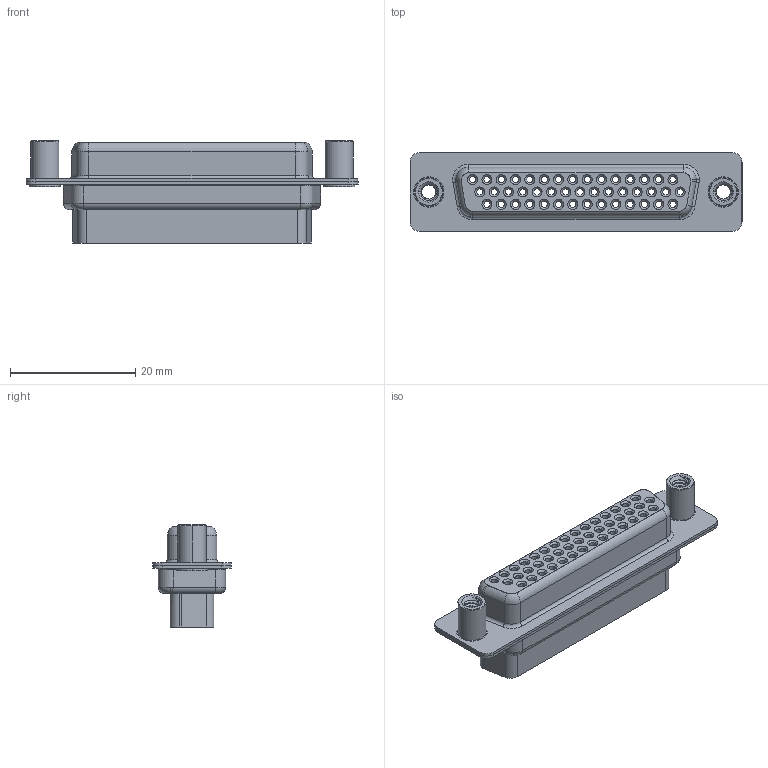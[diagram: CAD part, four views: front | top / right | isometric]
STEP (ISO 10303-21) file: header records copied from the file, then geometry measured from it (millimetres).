
FILE_DESCRIPTION (( 'STEP AP203' ), '1' );
FILE_NAME ('638-044-010-048.STEP', '2020-07-18T16:41:32', ( '' ), ( '' ), 'SwSTEP 2.0', 'SolidWorks 2020', '' );
FILE_SCHEMA (( 'CONFIG_CONTROL_DESIGN' ));
Length unit declared in the file: millimetre
Products named in the file (5): 638 Shell Rear_44 Contacts; 638 4-40 Threaded Standoff; 638 Housing_44 Contacts HP; 638-044-010-048; 638 Shell Front_44 Contacts
Assembly tree (5 placements, depth 2):
  638-044-010-048
    638 Housing_44 Contacts HP
    638 Shell Front_44 Contacts
    638 Shell Rear_44 Contacts
    638 4-40 Threaded Standoff  x2
Bounding box: 53.04 x 12.6 x 16.3 mm (x, y, z)
Volume: 3540.5 mm3; surface area: 9734.6 mm2
Topology: 5 solids, 5 shells, 885 faces, 2009 edges, 1279 vertices
Faces by surface type: cylinder 517, plane 201, cone 104, torus 57, bspline 6
Entity records: 26071 total; most frequent: CARTESIAN_POINT 5863, DIRECTION 4538, ORIENTED_EDGE 3764, AXIS2_PLACEMENT_3D 1917, EDGE_CURVE 1882, VERTEX_POINT 1197, EDGE_LOOP 1079, CIRCLE 1077
